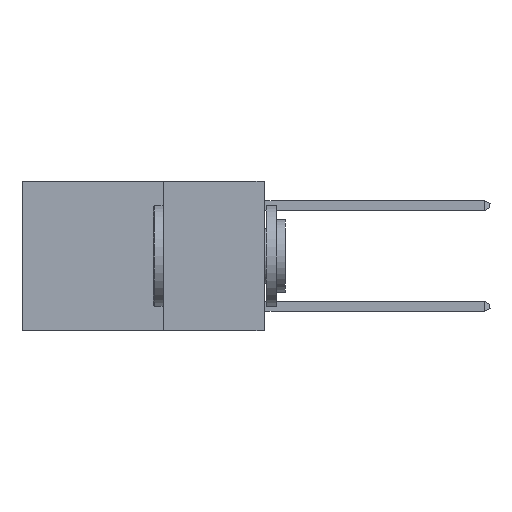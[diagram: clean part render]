
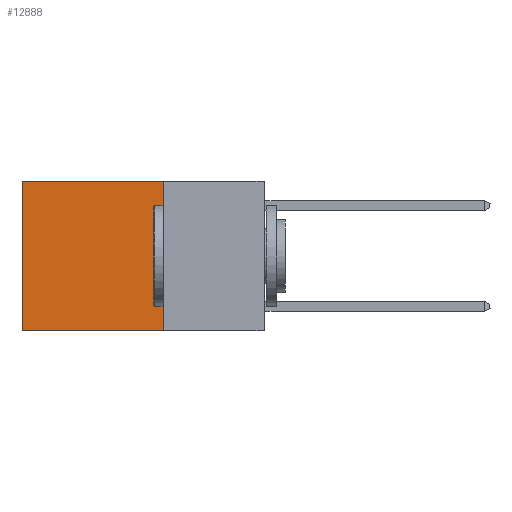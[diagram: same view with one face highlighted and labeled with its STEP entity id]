
A CAD part, left-side view. The second image highlights one B-rep face of the part: STEP entity #12888.
In plain terms, the highlighted planar face has unit normal (-1, 0, 0).
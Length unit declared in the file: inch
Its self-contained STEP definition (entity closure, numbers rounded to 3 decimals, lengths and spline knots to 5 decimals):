
#228 = CARTESIAN_POINT ( 'NONE',  ( 0.2625, 0.25, -0.37 ) ) ;
#434 = LINE ( 'NONE', #11229, #17148 ) ;
#709 = EDGE_CURVE ( 'NONE', #3398, #13701, #19929, .T. ) ;
#2203 = DIRECTION ( 'NONE',  ( 0., 0., -1. ) ) ;
#2289 = ORIENTED_EDGE ( 'NONE', *, *, #3093, .F. ) ;
#3080 = VECTOR ( 'NONE', #17293, 39.37008 ) ;
#3093 = EDGE_CURVE ( 'NONE', #17255, #13701, #15876, .T. ) ;
#3398 = VERTEX_POINT ( 'NONE', #7504 ) ;
#4695 = EDGE_CURVE ( 'NONE', #11104, #3398, #434, .T. ) ;
#5098 = LINE ( 'NONE', #6749, #8242 ) ;
#6083 = VECTOR ( 'NONE', #20026, 39.37008 ) ;
#6737 = DIRECTION ( 'NONE',  ( 0., 1., 0. ) ) ;
#6749 = CARTESIAN_POINT ( 'NONE',  ( 0.2625, 0.25, 0. ) ) ;
#7504 = CARTESIAN_POINT ( 'NONE',  ( 0.2625, 0.6, 0. ) ) ;
#8242 = VECTOR ( 'NONE', #12974, 39.37008 ) ;
#8560 = CARTESIAN_POINT ( 'NONE',  ( 0.2625, 0.25, 0. ) ) ;
#10095 = FACE_OUTER_BOUND ( 'NONE', #12144, .T. ) ;
#10492 = CARTESIAN_POINT ( 'NONE',  ( 0.2625, 0.25, 0. ) ) ;
#10595 = ORIENTED_EDGE ( 'NONE', *, *, #709, .T. ) ;
#11104 = VERTEX_POINT ( 'NONE', #10492 ) ;
#11229 = CARTESIAN_POINT ( 'NONE',  ( 0.2625, 0.25, 0. ) ) ;
#12068 = CARTESIAN_POINT ( 'NONE',  ( 0.2625, 0.6, 0. ) ) ;
#12144 = EDGE_LOOP ( 'NONE', ( #10595, #2289, #13107, #14023 ) ) ;
#12888 = ADVANCED_FACE ( 'NONE', ( #10095 ), #16306, .F. ) ;
#12974 = DIRECTION ( 'NONE',  ( 0., 0., -1. ) ) ;
#13107 = ORIENTED_EDGE ( 'NONE', *, *, #19889, .F. ) ;
#13701 = VERTEX_POINT ( 'NONE', #17668 ) ;
#14023 = ORIENTED_EDGE ( 'NONE', *, *, #4695, .T. ) ;
#14358 = CARTESIAN_POINT ( 'NONE',  ( 0.2625, 0.25, -0.37 ) ) ;
#14785 = DIRECTION ( 'NONE',  ( 1., 0., 0. ) ) ;
#15876 = LINE ( 'NONE', #14358, #3080 ) ;
#15887 = AXIS2_PLACEMENT_3D ( 'NONE', #8560, #14785, #2203 ) ;
#16306 = PLANE ( 'NONE',  #15887 ) ;
#17148 = VECTOR ( 'NONE', #6737, 39.37008 ) ;
#17255 = VERTEX_POINT ( 'NONE', #228 ) ;
#17293 = DIRECTION ( 'NONE',  ( 0., 1., 0. ) ) ;
#17668 = CARTESIAN_POINT ( 'NONE',  ( 0.2625, 0.6, -0.37 ) ) ;
#19889 = EDGE_CURVE ( 'NONE', #11104, #17255, #5098, .T. ) ;
#19929 = LINE ( 'NONE', #12068, #6083 ) ;
#20026 = DIRECTION ( 'NONE',  ( 0., 0., -1. ) ) ;
